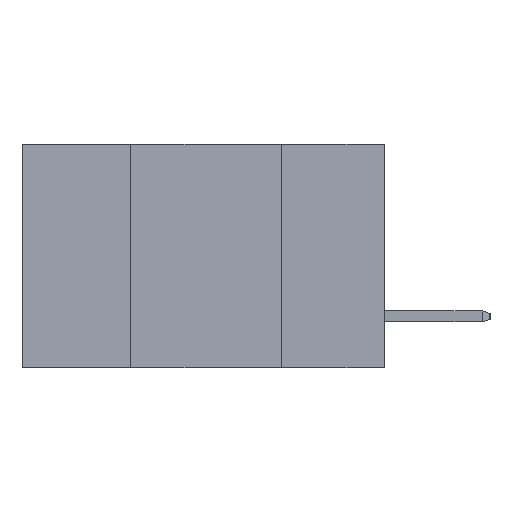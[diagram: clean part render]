
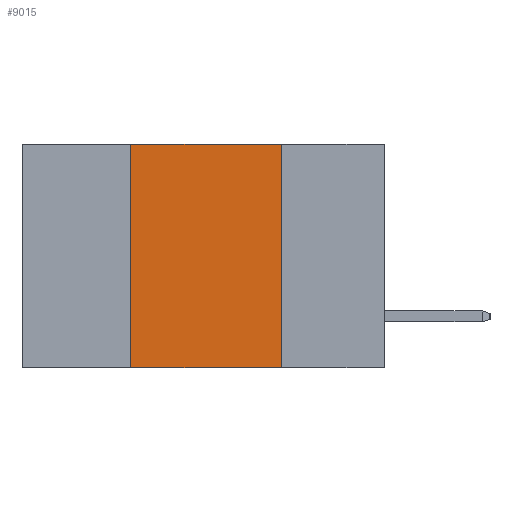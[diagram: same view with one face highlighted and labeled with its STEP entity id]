
A CAD part, left-side view. The second image highlights one B-rep face of the part: STEP entity #9015.
In plain terms, the highlighted planar face has unit normal (-1, 0, 0).
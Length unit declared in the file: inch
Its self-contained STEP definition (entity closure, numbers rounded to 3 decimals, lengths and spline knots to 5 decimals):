
#224 = VECTOR ( 'NONE', #7864, 39.37008 ) ;
#265 = DIRECTION ( 'NONE',  ( 0., -1., 0. ) ) ;
#418 = DIRECTION ( 'NONE',  ( 0., -1., 0. ) ) ;
#720 = EDGE_CURVE ( 'NONE', #7774, #11627, #9752, .T. ) ;
#789 = ORIENTED_EDGE ( 'NONE', *, *, #11068, .F. ) ;
#875 = CARTESIAN_POINT ( 'NONE',  ( 0., 0.42, 0. ) ) ;
#902 = VERTEX_POINT ( 'NONE', #6421 ) ;
#1157 = ORIENTED_EDGE ( 'NONE', *, *, #6484, .T. ) ;
#1206 = FACE_OUTER_BOUND ( 'NONE', #2324, .T. ) ;
#2324 = EDGE_LOOP ( 'NONE', ( #9279, #12644, #789, #1157 ) ) ;
#2611 = CARTESIAN_POINT ( 'NONE',  ( 0., 0.6, -0.37 ) ) ;
#3055 = CARTESIAN_POINT ( 'NONE',  ( 0., 0.17, -0.37 ) ) ;
#3738 = LINE ( 'NONE', #2611, #9820 ) ;
#4172 = PLANE ( 'NONE',  #4751 ) ;
#4751 = AXIS2_PLACEMENT_3D ( 'NONE', #13220, #13279, #6494 ) ;
#4926 = DIRECTION ( 'NONE',  ( 0., 0., -1. ) ) ;
#5179 = CARTESIAN_POINT ( 'NONE',  ( 0., 0.17, 0. ) ) ;
#6184 = CARTESIAN_POINT ( 'NONE',  ( 0., 0.6, 0. ) ) ;
#6421 = CARTESIAN_POINT ( 'NONE',  ( 0., 0.42, 0. ) ) ;
#6484 = EDGE_CURVE ( 'NONE', #8415, #11627, #3738, .T. ) ;
#6494 = DIRECTION ( 'NONE',  ( 0., 0., -1. ) ) ;
#6780 = VECTOR ( 'NONE', #4926, 39.37008 ) ;
#7774 = VERTEX_POINT ( 'NONE', #8768 ) ;
#7864 = DIRECTION ( 'NONE',  ( 0., 0., 1. ) ) ;
#8415 = VERTEX_POINT ( 'NONE', #12168 ) ;
#8768 = CARTESIAN_POINT ( 'NONE',  ( 0., 0.17, 0. ) ) ;
#9015 = ADVANCED_FACE ( 'NONE', ( #1206 ), #4172, .F. ) ;
#9279 = ORIENTED_EDGE ( 'NONE', *, *, #720, .F. ) ;
#9752 = LINE ( 'NONE', #5179, #6780 ) ;
#9820 = VECTOR ( 'NONE', #265, 39.37008 ) ;
#11068 = EDGE_CURVE ( 'NONE', #8415, #902, #12104, .T. ) ;
#11357 = VECTOR ( 'NONE', #418, 39.37008 ) ;
#11627 = VERTEX_POINT ( 'NONE', #3055 ) ;
#11698 = LINE ( 'NONE', #6184, #11357 ) ;
#12104 = LINE ( 'NONE', #875, #224 ) ;
#12168 = CARTESIAN_POINT ( 'NONE',  ( 0., 0.42, -0.37 ) ) ;
#12644 = ORIENTED_EDGE ( 'NONE', *, *, #13799, .F. ) ;
#13220 = CARTESIAN_POINT ( 'NONE',  ( 0., 0.6, 0. ) ) ;
#13279 = DIRECTION ( 'NONE',  ( 1., 0., 0. ) ) ;
#13799 = EDGE_CURVE ( 'NONE', #902, #7774, #11698, .T. ) ;
